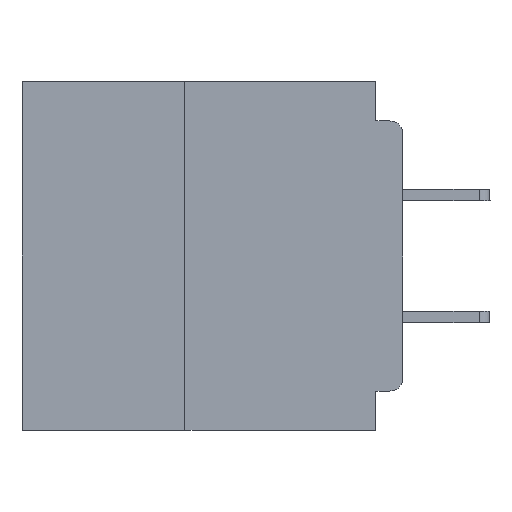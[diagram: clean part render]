
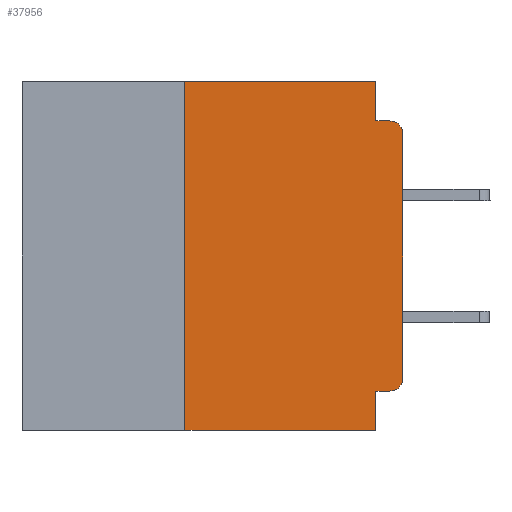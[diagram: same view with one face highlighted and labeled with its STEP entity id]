
A CAD part, left-side view. The second image highlights one B-rep face of the part: STEP entity #37956.
In plain terms, the highlighted planar face has unit normal (-1, 0, 0).
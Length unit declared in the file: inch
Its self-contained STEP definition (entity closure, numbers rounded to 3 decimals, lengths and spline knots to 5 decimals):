
#746 = CIRCLE ( 'NONE', #55975, 0.015 ) ;
#2123 = VERTEX_POINT ( 'NONE', #47276 ) ;
#2238 = CARTESIAN_POINT ( 'NONE',  ( 0., 0.031, -0.045 ) ) ;
#2654 = ORIENTED_EDGE ( 'NONE', *, *, #36425, .F. ) ;
#2954 = VERTEX_POINT ( 'NONE', #2238 ) ;
#3457 = LINE ( 'NONE', #50874, #42761 ) ;
#3617 = CARTESIAN_POINT ( 'NONE',  ( 0., 0.015, -0.06 ) ) ;
#4054 = LINE ( 'NONE', #14961, #12915 ) ;
#4824 = VECTOR ( 'NONE', #23450, 39.37008 ) ;
#4891 = CARTESIAN_POINT ( 'NONE',  ( 0., 0.437, 0. ) ) ;
#6013 = CARTESIAN_POINT ( 'NONE',  ( 0., 0.031, -0.355 ) ) ;
#6310 = CARTESIAN_POINT ( 'NONE',  ( 0., 0., 0. ) ) ;
#6807 = DIRECTION ( 'NONE',  ( 0., -1., 0. ) ) ;
#7981 = CARTESIAN_POINT ( 'NONE',  ( 0., 0.031, -0.4 ) ) ;
#8805 = DIRECTION ( 'NONE',  ( 0., 0., -1. ) ) ;
#9313 = VERTEX_POINT ( 'NONE', #34528 ) ;
#9858 = PLANE ( 'NONE',  #13197 ) ;
#10081 = DIRECTION ( 'NONE',  ( 1., 0., 0. ) ) ;
#10252 = CIRCLE ( 'NONE', #24315, 0.015 ) ;
#12344 = EDGE_CURVE ( 'NONE', #30539, #2123, #65167, .T. ) ;
#12915 = VECTOR ( 'NONE', #45800, 39.37008 ) ;
#13057 = ORIENTED_EDGE ( 'NONE', *, *, #47497, .F. ) ;
#13197 = AXIS2_PLACEMENT_3D ( 'NONE', #4891, #10081, #45881 ) ;
#13229 = VECTOR ( 'NONE', #26175, 39.37008 ) ;
#14276 = ORIENTED_EDGE ( 'NONE', *, *, #12344, .T. ) ;
#14961 = CARTESIAN_POINT ( 'NONE',  ( 0., 0.437, -0.4 ) ) ;
#19726 = ORIENTED_EDGE ( 'NONE', *, *, #41663, .F. ) ;
#20126 = LINE ( 'NONE', #33776, #4824 ) ;
#20500 = CARTESIAN_POINT ( 'NONE',  ( 0., 0.031, 0. ) ) ;
#22613 = CARTESIAN_POINT ( 'NONE',  ( 0., 0.015, -0.34 ) ) ;
#23450 = DIRECTION ( 'NONE',  ( 0., 1., 0. ) ) ;
#23844 = LINE ( 'NONE', #20500, #35887 ) ;
#24315 = AXIS2_PLACEMENT_3D ( 'NONE', #22613, #58295, #27790 ) ;
#24319 = EDGE_CURVE ( 'NONE', #39660, #30539, #10252, .T. ) ;
#25191 = EDGE_CURVE ( 'NONE', #2123, #35303, #746, .T. ) ;
#26175 = DIRECTION ( 'NONE',  ( 0., 0., 1. ) ) ;
#27790 = DIRECTION ( 'NONE',  ( 0., 0., -1. ) ) ;
#28466 = ORIENTED_EDGE ( 'NONE', *, *, #38560, .T. ) ;
#28986 = CARTESIAN_POINT ( 'NONE',  ( 0., 0.015, -0.355 ) ) ;
#29899 = ORIENTED_EDGE ( 'NONE', *, *, #36910, .F. ) ;
#30539 = VERTEX_POINT ( 'NONE', #61722 ) ;
#33776 = CARTESIAN_POINT ( 'NONE',  ( 0., 0., -0.355 ) ) ;
#34528 = CARTESIAN_POINT ( 'NONE',  ( 0., 0.25, -0.4 ) ) ;
#35157 = ORIENTED_EDGE ( 'NONE', *, *, #48072, .F. ) ;
#35303 = VERTEX_POINT ( 'NONE', #42379 ) ;
#35887 = VECTOR ( 'NONE', #40843, 39.37008 ) ;
#36425 = EDGE_CURVE ( 'NONE', #37629, #63637, #54261, .T. ) ;
#36910 = EDGE_CURVE ( 'NONE', #43985, #2954, #23844, .T. ) ;
#37282 = VERTEX_POINT ( 'NONE', #53741 ) ;
#37292 = DIRECTION ( 'NONE',  ( 0., 0., 1. ) ) ;
#37629 = VERTEX_POINT ( 'NONE', #6013 ) ;
#37956 = ADVANCED_FACE ( 'NONE', ( #63353 ), #9858, .F. ) ;
#38167 = ORIENTED_EDGE ( 'NONE', *, *, #24319, .T. ) ;
#38560 = EDGE_CURVE ( 'NONE', #9313, #63637, #4054, .T. ) ;
#39506 = DIRECTION ( 'NONE',  ( -1., 0., 0. ) ) ;
#39660 = VERTEX_POINT ( 'NONE', #28986 ) ;
#39728 = LINE ( 'NONE', #47763, #51685 ) ;
#40843 = DIRECTION ( 'NONE',  ( 0., 0., -1. ) ) ;
#41253 = VECTOR ( 'NONE', #37292, 39.37008 ) ;
#41663 = EDGE_CURVE ( 'NONE', #37282, #43985, #39728, .T. ) ;
#42379 = CARTESIAN_POINT ( 'NONE',  ( 0., 0.015, -0.045 ) ) ;
#42761 = VECTOR ( 'NONE', #55983, 39.37008 ) ;
#43985 = VERTEX_POINT ( 'NONE', #48552 ) ;
#45800 = DIRECTION ( 'NONE',  ( 0., -1., 0. ) ) ;
#45881 = DIRECTION ( 'NONE',  ( 0., 0., -1. ) ) ;
#47276 = CARTESIAN_POINT ( 'NONE',  ( 0., 0., -0.06 ) ) ;
#47497 = EDGE_CURVE ( 'NONE', #9313, #37282, #55585, .T. ) ;
#47763 = CARTESIAN_POINT ( 'NONE',  ( 0., 0.437, 0. ) ) ;
#48072 = EDGE_CURVE ( 'NONE', #2954, #35303, #3457, .T. ) ;
#48552 = CARTESIAN_POINT ( 'NONE',  ( 0., 0.031, 0. ) ) ;
#50874 = CARTESIAN_POINT ( 'NONE',  ( 0., 0., -0.045 ) ) ;
#51616 = CARTESIAN_POINT ( 'NONE',  ( 0., 0.25, -0.4 ) ) ;
#51685 = VECTOR ( 'NONE', #6807, 39.37008 ) ;
#52272 = CARTESIAN_POINT ( 'NONE',  ( 0., 0.031, -0.4 ) ) ;
#53741 = CARTESIAN_POINT ( 'NONE',  ( 0., 0.25, 0. ) ) ;
#54261 = LINE ( 'NONE', #52272, #66203 ) ;
#55585 = LINE ( 'NONE', #51616, #13229 ) ;
#55975 = AXIS2_PLACEMENT_3D ( 'NONE', #3617, #39506, #8805 ) ;
#55983 = DIRECTION ( 'NONE',  ( 0., -1., 0. ) ) ;
#56849 = EDGE_CURVE ( 'NONE', #39660, #37629, #20126, .T. ) ;
#58295 = DIRECTION ( 'NONE',  ( -1., 0., 0. ) ) ;
#61722 = CARTESIAN_POINT ( 'NONE',  ( 0., 0., -0.34 ) ) ;
#62278 = DIRECTION ( 'NONE',  ( 0., 0., -1. ) ) ;
#62911 = ORIENTED_EDGE ( 'NONE', *, *, #56849, .F. ) ;
#63353 = FACE_OUTER_BOUND ( 'NONE', #65993, .T. ) ;
#63637 = VERTEX_POINT ( 'NONE', #7981 ) ;
#64015 = ORIENTED_EDGE ( 'NONE', *, *, #25191, .T. ) ;
#65167 = LINE ( 'NONE', #6310, #41253 ) ;
#65993 = EDGE_LOOP ( 'NONE', ( #14276, #64015, #35157, #29899, #19726, #13057, #28466, #2654, #62911, #38167 ) ) ;
#66203 = VECTOR ( 'NONE', #62278, 39.37008 ) ;
